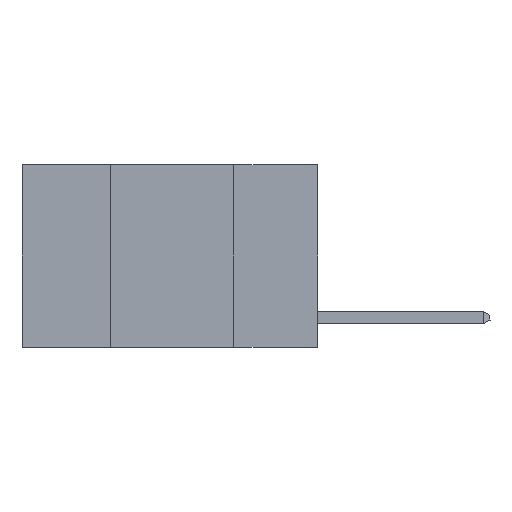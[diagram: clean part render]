
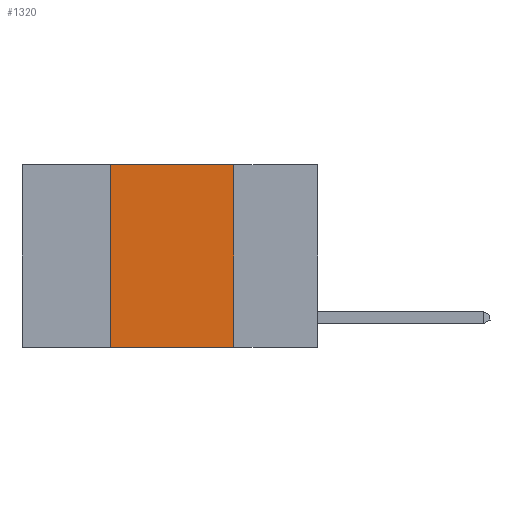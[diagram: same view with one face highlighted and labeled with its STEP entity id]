
A CAD part, left-side view. The second image highlights one B-rep face of the part: STEP entity #1320.
In plain terms, the highlighted planar face has unit normal (-1, 0, 0).
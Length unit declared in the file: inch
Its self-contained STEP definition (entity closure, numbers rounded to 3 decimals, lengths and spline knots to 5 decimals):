
#24 = LINE ( 'NONE', #8851, #1900 ) ;
#334 = ORIENTED_EDGE ( 'NONE', *, *, #3993, .F. ) ;
#628 = ORIENTED_EDGE ( 'NONE', *, *, #9849, .F. ) ;
#1120 = DIRECTION ( 'NONE',  ( 0., 0., 1. ) ) ;
#1138 = VERTEX_POINT ( 'NONE', #4382 ) ;
#1167 = DIRECTION ( 'NONE',  ( 0., 0., -1. ) ) ;
#1320 = ADVANCED_FACE ( 'NONE', ( #8504 ), #7394, .F. ) ;
#1900 = VECTOR ( 'NONE', #4984, 39.37008 ) ;
#2028 = DIRECTION ( 'NONE',  ( 0., -1., 0. ) ) ;
#2803 = ORIENTED_EDGE ( 'NONE', *, *, #5833, .T. ) ;
#2837 = VERTEX_POINT ( 'NONE', #5365 ) ;
#2848 = VECTOR ( 'NONE', #1167, 39.37008 ) ;
#3202 = LINE ( 'NONE', #8813, #7029 ) ;
#3993 = EDGE_CURVE ( 'NONE', #2837, #5665, #4849, .T. ) ;
#4055 = CARTESIAN_POINT ( 'NONE',  ( 0., 0.17, -0.37 ) ) ;
#4382 = CARTESIAN_POINT ( 'NONE',  ( 0., 0.42, 0. ) ) ;
#4474 = VERTEX_POINT ( 'NONE', #4838 ) ;
#4553 = ORIENTED_EDGE ( 'NONE', *, *, #7476, .F. ) ;
#4838 = CARTESIAN_POINT ( 'NONE',  ( 0., 0.42, -0.37 ) ) ;
#4849 = LINE ( 'NONE', #5770, #2848 ) ;
#4984 = DIRECTION ( 'NONE',  ( 0., -1., 0. ) ) ;
#5365 = CARTESIAN_POINT ( 'NONE',  ( 0., 0.17, 0. ) ) ;
#5651 = DIRECTION ( 'NONE',  ( 0., 0., -1. ) ) ;
#5665 = VERTEX_POINT ( 'NONE', #4055 ) ;
#5770 = CARTESIAN_POINT ( 'NONE',  ( 0., 0.17, 0. ) ) ;
#5794 = CARTESIAN_POINT ( 'NONE',  ( 0., 0.6, -0.37 ) ) ;
#5833 = EDGE_CURVE ( 'NONE', #4474, #5665, #6365, .T. ) ;
#5920 = VECTOR ( 'NONE', #2028, 39.37008 ) ;
#6365 = LINE ( 'NONE', #5794, #5920 ) ;
#7029 = VECTOR ( 'NONE', #1120, 39.37008 ) ;
#7318 = EDGE_LOOP ( 'NONE', ( #334, #4553, #628, #2803 ) ) ;
#7394 = PLANE ( 'NONE',  #8669 ) ;
#7476 = EDGE_CURVE ( 'NONE', #1138, #2837, #24, .T. ) ;
#7526 = CARTESIAN_POINT ( 'NONE',  ( 0., 0.6, 0. ) ) ;
#8504 = FACE_OUTER_BOUND ( 'NONE', #7318, .T. ) ;
#8669 = AXIS2_PLACEMENT_3D ( 'NONE', #7526, #8932, #5651 ) ;
#8813 = CARTESIAN_POINT ( 'NONE',  ( 0., 0.42, 0. ) ) ;
#8851 = CARTESIAN_POINT ( 'NONE',  ( 0., 0.6, 0. ) ) ;
#8932 = DIRECTION ( 'NONE',  ( 1., 0., 0. ) ) ;
#9849 = EDGE_CURVE ( 'NONE', #4474, #1138, #3202, .T. ) ;
